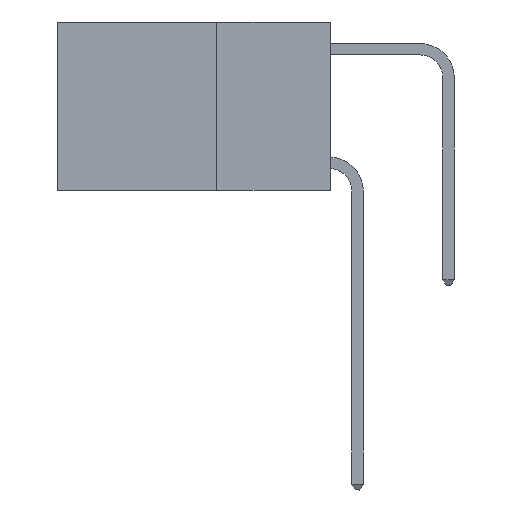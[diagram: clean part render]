
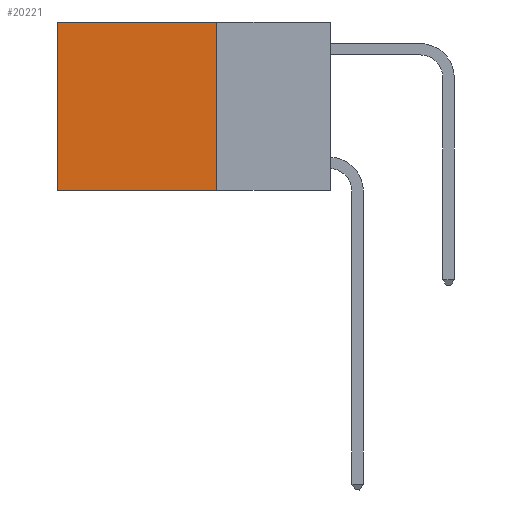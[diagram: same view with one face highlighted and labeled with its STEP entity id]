
A CAD part, left-side view. The second image highlights one B-rep face of the part: STEP entity #20221.
In plain terms, the highlighted planar face has unit normal (-1, 0, 0).
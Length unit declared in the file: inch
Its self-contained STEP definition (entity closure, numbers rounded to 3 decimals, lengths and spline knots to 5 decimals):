
#28 = VECTOR ( 'NONE', #31912, 39.37008 ) ;
#134 = VECTOR ( 'NONE', #4474, 39.37008 ) ;
#1700 = DIRECTION ( 'NONE',  ( 0., 0., -1. ) ) ;
#3622 = EDGE_CURVE ( 'NONE', #8459, #11977, #31411, .T. ) ;
#4474 = DIRECTION ( 'NONE',  ( 0., 1., 0. ) ) ;
#5130 = DIRECTION ( 'NONE',  ( 1., 0., 0. ) ) ;
#6358 = CARTESIAN_POINT ( 'NONE',  ( 0.2625, 0.25, 0. ) ) ;
#7158 = CARTESIAN_POINT ( 'NONE',  ( 0.2625, 0.25, 0. ) ) ;
#8358 = VERTEX_POINT ( 'NONE', #26149 ) ;
#8459 = VERTEX_POINT ( 'NONE', #6358 ) ;
#8704 = EDGE_CURVE ( 'NONE', #8459, #8358, #19904, .T. ) ;
#10908 = LINE ( 'NONE', #16856, #11709 ) ;
#11709 = VECTOR ( 'NONE', #1700, 39.37008 ) ;
#11977 = VERTEX_POINT ( 'NONE', #26700 ) ;
#16856 = CARTESIAN_POINT ( 'NONE',  ( 0.2625, 0.6, 0. ) ) ;
#17526 = DIRECTION ( 'NONE',  ( 0., 0., -1. ) ) ;
#17744 = PLANE ( 'NONE',  #25210 ) ;
#18778 = FACE_OUTER_BOUND ( 'NONE', #19940, .T. ) ;
#18874 = ORIENTED_EDGE ( 'NONE', *, *, #3622, .F. ) ;
#19026 = DIRECTION ( 'NONE',  ( 0., 0., -1. ) ) ;
#19904 = LINE ( 'NONE', #7158, #134 ) ;
#19940 = EDGE_LOOP ( 'NONE', ( #24388, #30021, #18874, #31048 ) ) ;
#20221 = ADVANCED_FACE ( 'NONE', ( #18778 ), #17744, .F. ) ;
#20276 = CARTESIAN_POINT ( 'NONE',  ( 0.2625, 0.25, 0. ) ) ;
#22134 = LINE ( 'NONE', #26614, #28 ) ;
#24388 = ORIENTED_EDGE ( 'NONE', *, *, #32343, .T. ) ;
#25210 = AXIS2_PLACEMENT_3D ( 'NONE', #20276, #5130, #17526 ) ;
#26149 = CARTESIAN_POINT ( 'NONE',  ( 0.2625, 0.6, 0. ) ) ;
#26560 = CARTESIAN_POINT ( 'NONE',  ( 0.2625, 0.25, 0. ) ) ;
#26614 = CARTESIAN_POINT ( 'NONE',  ( 0.2625, 0.25, -0.37 ) ) ;
#26700 = CARTESIAN_POINT ( 'NONE',  ( 0.2625, 0.25, -0.37 ) ) ;
#27045 = CARTESIAN_POINT ( 'NONE',  ( 0.2625, 0.6, -0.37 ) ) ;
#30021 = ORIENTED_EDGE ( 'NONE', *, *, #30181, .F. ) ;
#30181 = EDGE_CURVE ( 'NONE', #11977, #30713, #22134, .T. ) ;
#30606 = VECTOR ( 'NONE', #19026, 39.37008 ) ;
#30713 = VERTEX_POINT ( 'NONE', #27045 ) ;
#31048 = ORIENTED_EDGE ( 'NONE', *, *, #8704, .T. ) ;
#31411 = LINE ( 'NONE', #26560, #30606 ) ;
#31912 = DIRECTION ( 'NONE',  ( 0., 1., 0. ) ) ;
#32343 = EDGE_CURVE ( 'NONE', #8358, #30713, #10908, .T. ) ;
